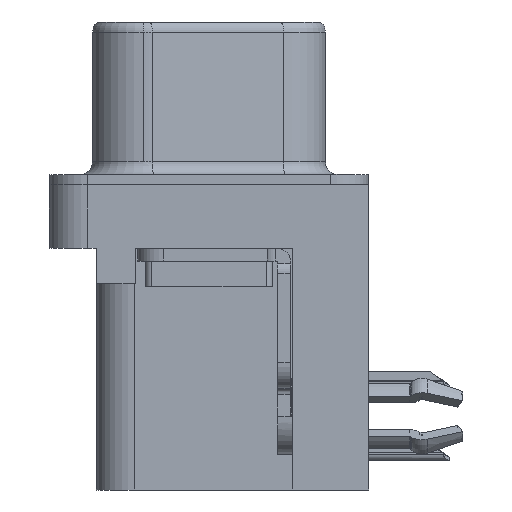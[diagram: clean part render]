
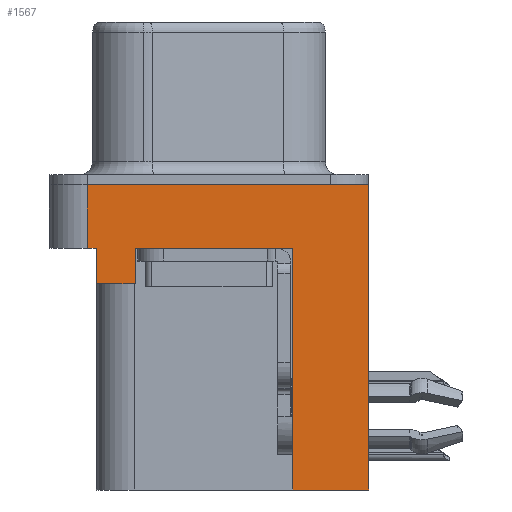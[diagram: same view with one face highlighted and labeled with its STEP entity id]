
A CAD part, left-side view. The second image highlights one B-rep face of the part: STEP entity #1567.
In plain terms, the highlighted planar face has unit normal (-1, 0, 0).
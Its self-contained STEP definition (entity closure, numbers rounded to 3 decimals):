
#204 = VECTOR ( 'NONE', #13111, 1000. ) ;
#290 = DIRECTION ( 'NONE',  ( 0., 1., 0. ) ) ;
#381 = LINE ( 'NONE', #26283, #16108 ) ;
#424 = VECTOR ( 'NONE', #290, 1000. ) ;
#681 = CARTESIAN_POINT ( 'NONE',  ( -2.91, -6.275, -2.5 ) ) ;
#1059 = ORIENTED_EDGE ( 'NONE', *, *, #25215, .F. ) ;
#1300 = LINE ( 'NONE', #18204, #15770 ) ;
#1567 = ADVANCED_FACE ( 'NONE', ( #14052 ), #12071, .T. ) ;
#1783 = ORIENTED_EDGE ( 'NONE', *, *, #2695, .T. ) ;
#1881 = LINE ( 'NONE', #22492, #24931 ) ;
#2695 = EDGE_CURVE ( 'NONE', #25897, #2866, #7208, .T. ) ;
#2866 = VERTEX_POINT ( 'NONE', #26374 ) ;
#3817 = CARTESIAN_POINT ( 'NONE',  ( -2.91, 4.775, -2.5 ) ) ;
#4689 = VERTEX_POINT ( 'NONE', #7848 ) ;
#5513 = LINE ( 'NONE', #7697, #424 ) ;
#5831 = VERTEX_POINT ( 'NONE', #18000 ) ;
#6395 = ORIENTED_EDGE ( 'NONE', *, *, #15488, .T. ) ;
#6873 = VECTOR ( 'NONE', #24067, 1000. ) ;
#6973 = VECTOR ( 'NONE', #10723, 1000. ) ;
#6979 = ORIENTED_EDGE ( 'NONE', *, *, #9996, .F. ) ;
#6984 = ORIENTED_EDGE ( 'NONE', *, *, #8678, .F. ) ;
#7208 = LINE ( 'NONE', #9028, #18079 ) ;
#7697 = CARTESIAN_POINT ( 'NONE',  ( -2.91, 4.425, -3.9 ) ) ;
#7848 = CARTESIAN_POINT ( 'NONE',  ( -2.91, 4.425, -2.5 ) ) ;
#8279 = ORIENTED_EDGE ( 'NONE', *, *, #9789, .F. ) ;
#8678 = EDGE_CURVE ( 'NONE', #13227, #19877, #1300, .T. ) ;
#8792 = EDGE_CURVE ( 'NONE', #12387, #4689, #381, .T. ) ;
#9028 = CARTESIAN_POINT ( 'NONE',  ( -2.91, 2.895, -3.9 ) ) ;
#9203 = CARTESIAN_POINT ( 'NONE',  ( -2.91, -3.295, -12. ) ) ;
#9764 = CARTESIAN_POINT ( 'NONE',  ( -2.91, 2.895, -3.9 ) ) ;
#9789 = EDGE_CURVE ( 'NONE', #15864, #10659, #1881, .T. ) ;
#9996 = EDGE_CURVE ( 'NONE', #25897, #20658, #5513, .T. ) ;
#10014 = ORIENTED_EDGE ( 'NONE', *, *, #8792, .T. ) ;
#10445 = VECTOR ( 'NONE', #10878, 1000. ) ;
#10471 = CARTESIAN_POINT ( 'NONE',  ( -2.91, -6.275, -2.5 ) ) ;
#10508 = LINE ( 'NONE', #681, #204 ) ;
#10659 = VERTEX_POINT ( 'NONE', #25890 ) ;
#10723 = DIRECTION ( 'NONE',  ( 0., 1., 0. ) ) ;
#10843 = CARTESIAN_POINT ( 'NONE',  ( -2.91, 4.425, -3.9 ) ) ;
#10878 = DIRECTION ( 'NONE',  ( 0., 0., 1. ) ) ;
#11201 = EDGE_CURVE ( 'NONE', #2866, #19877, #10508, .T. ) ;
#12071 = PLANE ( 'NONE',  #18822 ) ;
#12387 = VERTEX_POINT ( 'NONE', #18525 ) ;
#12524 = CARTESIAN_POINT ( 'NONE',  ( -2.91, 4.775, 0. ) ) ;
#13111 = DIRECTION ( 'NONE',  ( 0., -1., 0. ) ) ;
#13227 = VERTEX_POINT ( 'NONE', #9203 ) ;
#13943 = LINE ( 'NONE', #10471, #16465 ) ;
#13987 = LINE ( 'NONE', #22944, #10445 ) ;
#14052 = FACE_OUTER_BOUND ( 'NONE', #22680, .T. ) ;
#14824 = ORIENTED_EDGE ( 'NONE', *, *, #21114, .F. ) ;
#15488 = EDGE_CURVE ( 'NONE', #5831, #10659, #13943, .T. ) ;
#15770 = VECTOR ( 'NONE', #18458, 1000. ) ;
#15864 = VERTEX_POINT ( 'NONE', #12524 ) ;
#16108 = VECTOR ( 'NONE', #20177, 1000. ) ;
#16465 = VECTOR ( 'NONE', #24742, 1000. ) ;
#16606 = CARTESIAN_POINT ( 'NONE',  ( -2.91, -3.295, -12. ) ) ;
#17612 = DIRECTION ( 'NONE',  ( 0., 0., 1. ) ) ;
#18000 = CARTESIAN_POINT ( 'NONE',  ( -2.91, -6.275, -12. ) ) ;
#18079 = VECTOR ( 'NONE', #17612, 1000. ) ;
#18204 = CARTESIAN_POINT ( 'NONE',  ( -2.91, -3.295, -12. ) ) ;
#18367 = CARTESIAN_POINT ( 'NONE',  ( -2.91, -3.295, -2.5 ) ) ;
#18458 = DIRECTION ( 'NONE',  ( 0., 0., 1. ) ) ;
#18525 = CARTESIAN_POINT ( 'NONE',  ( -2.91, 4.775, -2.5 ) ) ;
#18822 = AXIS2_PLACEMENT_3D ( 'NONE', #25982, #19886, #22228 ) ;
#19877 = VERTEX_POINT ( 'NONE', #18367 ) ;
#19886 = DIRECTION ( 'NONE',  ( -1., 0., 0. ) ) ;
#20177 = DIRECTION ( 'NONE',  ( 0., -1., 0. ) ) ;
#20587 = DIRECTION ( 'NONE',  ( 0., -1., 0. ) ) ;
#20658 = VERTEX_POINT ( 'NONE', #10843 ) ;
#21046 = LINE ( 'NONE', #16606, #6973 ) ;
#21114 = EDGE_CURVE ( 'NONE', #5831, #13227, #21046, .T. ) ;
#22228 = DIRECTION ( 'NONE',  ( 0., 0., 1. ) ) ;
#22245 = ORIENTED_EDGE ( 'NONE', *, *, #25784, .F. ) ;
#22492 = CARTESIAN_POINT ( 'NONE',  ( -2.91, -6.275, 0. ) ) ;
#22680 = EDGE_LOOP ( 'NONE', ( #8279, #22245, #10014, #1059, #6979, #1783, #26125, #6984, #14824, #6395 ) ) ;
#22944 = CARTESIAN_POINT ( 'NONE',  ( -2.91, 4.425, -3.9 ) ) ;
#24067 = DIRECTION ( 'NONE',  ( 0., 0., 1. ) ) ;
#24742 = DIRECTION ( 'NONE',  ( 0., 0., 1. ) ) ;
#24931 = VECTOR ( 'NONE', #20587, 1000. ) ;
#25215 = EDGE_CURVE ( 'NONE', #20658, #4689, #13987, .T. ) ;
#25758 = LINE ( 'NONE', #3817, #6873 ) ;
#25784 = EDGE_CURVE ( 'NONE', #12387, #15864, #25758, .T. ) ;
#25890 = CARTESIAN_POINT ( 'NONE',  ( -2.91, -6.275, 0. ) ) ;
#25897 = VERTEX_POINT ( 'NONE', #9764 ) ;
#25982 = CARTESIAN_POINT ( 'NONE',  ( -2.91, -6.275, -2.5 ) ) ;
#26125 = ORIENTED_EDGE ( 'NONE', *, *, #11201, .T. ) ;
#26283 = CARTESIAN_POINT ( 'NONE',  ( -2.91, -6.275, -2.5 ) ) ;
#26374 = CARTESIAN_POINT ( 'NONE',  ( -2.91, 2.895, -2.5 ) ) ;
